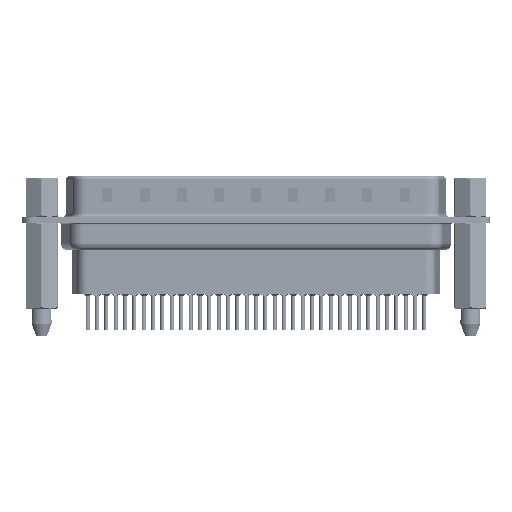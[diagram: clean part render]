
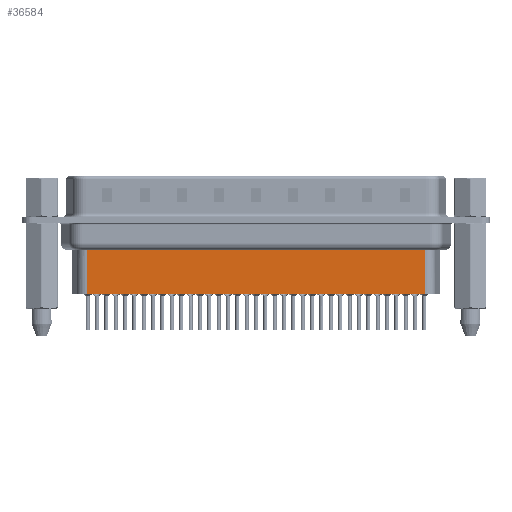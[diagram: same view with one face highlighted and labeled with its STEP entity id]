
A CAD part, front view. The second image highlights one B-rep face of the part: STEP entity #36584.
In plain terms, the highlighted planar face has unit normal (0, -1, 0).
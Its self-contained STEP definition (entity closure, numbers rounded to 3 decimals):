
#2589 = AXIS2_PLACEMENT_3D ( 'NONE', #7213, #30059, #15820 ) ;
#3098 = ORIENTED_EDGE ( 'NONE', *, *, #21591, .F. ) ;
#3776 = VECTOR ( 'NONE', #22396, 1000. ) ;
#4526 = DIRECTION ( 'NONE',  ( -1., 0., 0. ) ) ;
#7213 = CARTESIAN_POINT ( 'NONE',  ( 6.706, -3.5, -3.1 ) ) ;
#8178 = DIRECTION ( 'NONE',  ( -1., 0., 0. ) ) ;
#8210 = EDGE_LOOP ( 'NONE', ( #3098, #32239, #10045, #22107 ) ) ;
#10045 = ORIENTED_EDGE ( 'NONE', *, *, #17617, .T. ) ;
#13215 = LINE ( 'NONE', #33613, #3776 ) ;
#14337 = CARTESIAN_POINT ( 'NONE',  ( 6.459, -3.5, -4.097 ) ) ;
#15820 = DIRECTION ( 'NONE',  ( 1., 0., 0. ) ) ;
#16677 = VECTOR ( 'NONE', #4526, 1000. ) ;
#17617 = EDGE_CURVE ( 'NONE', #36974, #21646, #13215, .T. ) ;
#17655 = CARTESIAN_POINT ( 'NONE',  ( 56.794, -3.5, -3.1 ) ) ;
#18171 = VECTOR ( 'NONE', #8178, 1000. ) ;
#19573 = LINE ( 'NONE', #14337, #18171 ) ;
#20234 = CARTESIAN_POINT ( 'NONE',  ( 56.794, -3.5, -4.097 ) ) ;
#20390 = VERTEX_POINT ( 'NONE', #20234 ) ;
#20500 = EDGE_CURVE ( 'NONE', #28452, #21646, #30163, .T. ) ;
#21032 = CARTESIAN_POINT ( 'NONE',  ( 6.706, -3.5, -10.95 ) ) ;
#21443 = PLANE ( 'NONE',  #2589 ) ;
#21591 = EDGE_CURVE ( 'NONE', #20390, #28452, #33994, .T. ) ;
#21646 = VERTEX_POINT ( 'NONE', #21032 ) ;
#22107 = ORIENTED_EDGE ( 'NONE', *, *, #20500, .F. ) ;
#22396 = DIRECTION ( 'NONE',  ( 0., 0., -1. ) ) ;
#24251 = FACE_OUTER_BOUND ( 'NONE', #8210, .T. ) ;
#26440 = CARTESIAN_POINT ( 'NONE',  ( 56.794, -3.5, -10.95 ) ) ;
#26933 = VECTOR ( 'NONE', #28730, 1000. ) ;
#27163 = CARTESIAN_POINT ( 'NONE',  ( 6.706, -3.5, -10.95 ) ) ;
#27513 = EDGE_CURVE ( 'NONE', #20390, #36974, #19573, .T. ) ;
#28452 = VERTEX_POINT ( 'NONE', #26440 ) ;
#28730 = DIRECTION ( 'NONE',  ( 0., 0., -1. ) ) ;
#29693 = CARTESIAN_POINT ( 'NONE',  ( 6.706, -3.5, -4.097 ) ) ;
#30059 = DIRECTION ( 'NONE',  ( 0., -1., 0. ) ) ;
#30163 = LINE ( 'NONE', #27163, #16677 ) ;
#32239 = ORIENTED_EDGE ( 'NONE', *, *, #27513, .T. ) ;
#33613 = CARTESIAN_POINT ( 'NONE',  ( 6.706, -3.5, -3.1 ) ) ;
#33994 = LINE ( 'NONE', #17655, #26933 ) ;
#36584 = ADVANCED_FACE ( 'NONE', ( #24251 ), #21443, .T. ) ;
#36974 = VERTEX_POINT ( 'NONE', #29693 ) ;
